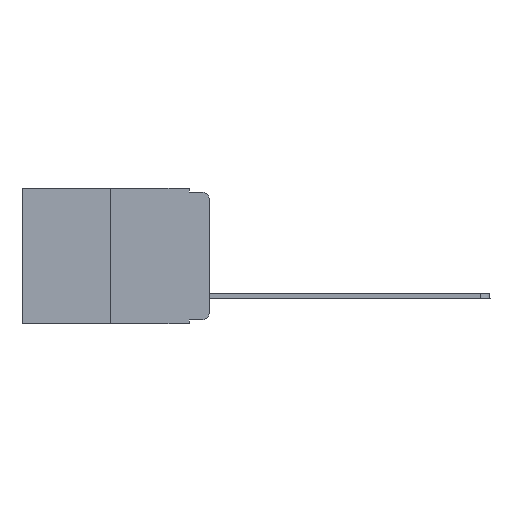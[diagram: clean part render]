
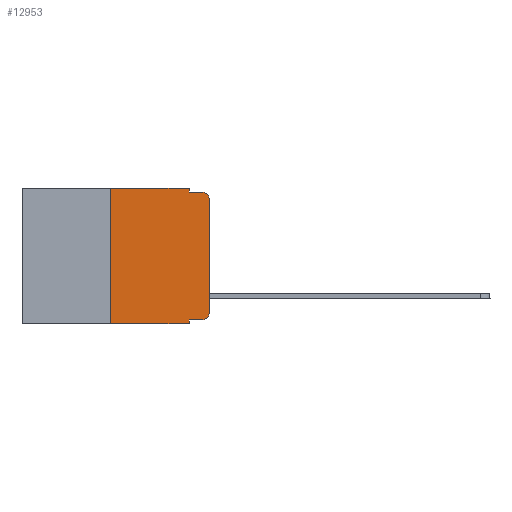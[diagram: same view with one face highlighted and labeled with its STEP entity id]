
A CAD part, left-side view. The second image highlights one B-rep face of the part: STEP entity #12953.
In plain terms, the highlighted planar face has unit normal (-1, 0, 0).
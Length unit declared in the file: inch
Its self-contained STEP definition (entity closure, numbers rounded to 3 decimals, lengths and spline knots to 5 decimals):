
#369 = ORIENTED_EDGE ( 'NONE', *, *, #9170, .F. ) ;
#787 = DIRECTION ( 'NONE',  ( 0., 0., -1. ) ) ;
#1045 = VECTOR ( 'NONE', #8616, 39.37008 ) ;
#1220 = ORIENTED_EDGE ( 'NONE', *, *, #12271, .F. ) ;
#1303 = CARTESIAN_POINT ( 'NONE',  ( 0., 0.02, -0.333 ) ) ;
#1340 = ORIENTED_EDGE ( 'NONE', *, *, #8053, .T. ) ;
#1372 = VERTEX_POINT ( 'NONE', #7355 ) ;
#1584 = CARTESIAN_POINT ( 'NONE',  ( 0., 0.051, 0. ) ) ;
#1749 = DIRECTION ( 'NONE',  ( 0., 0., 1. ) ) ;
#1909 = EDGE_CURVE ( 'NONE', #9740, #6897, #2141, .T. ) ;
#2013 = VERTEX_POINT ( 'NONE', #8496 ) ;
#2141 = LINE ( 'NONE', #3742, #11521 ) ;
#2171 = DIRECTION ( 'NONE',  ( 0., 0., -1. ) ) ;
#2292 = ORIENTED_EDGE ( 'NONE', *, *, #4062, .T. ) ;
#2533 = VECTOR ( 'NONE', #6343, 39.37008 ) ;
#2651 = DIRECTION ( 'NONE',  ( -1., 0., 0. ) ) ;
#2706 = CARTESIAN_POINT ( 'NONE',  ( 0., 0.02, -0.313 ) ) ;
#2746 = VERTEX_POINT ( 'NONE', #13359 ) ;
#2886 = CARTESIAN_POINT ( 'NONE',  ( 0., 0.02, -0.03 ) ) ;
#2942 = LINE ( 'NONE', #5876, #11788 ) ;
#3375 = AXIS2_PLACEMENT_3D ( 'NONE', #2706, #2651, #3918 ) ;
#3420 = AXIS2_PLACEMENT_3D ( 'NONE', #2886, #5226, #787 ) ;
#3734 = VECTOR ( 'NONE', #5573, 39.37008 ) ;
#3742 = CARTESIAN_POINT ( 'NONE',  ( 0., 0.051, 0. ) ) ;
#3799 = DIRECTION ( 'NONE',  ( 0., 0., -1. ) ) ;
#3918 = DIRECTION ( 'NONE',  ( 0., 0., -1. ) ) ;
#4062 = EDGE_CURVE ( 'NONE', #14175, #13535, #10064, .T. ) ;
#4861 = CARTESIAN_POINT ( 'NONE',  ( 0., 0.051, -0.01 ) ) ;
#5122 = VERTEX_POINT ( 'NONE', #8441 ) ;
#5226 = DIRECTION ( 'NONE',  ( -1., 0., 0. ) ) ;
#5497 = LINE ( 'NONE', #12083, #2533 ) ;
#5573 = DIRECTION ( 'NONE',  ( 0., 0., -1. ) ) ;
#5605 = VECTOR ( 'NONE', #13999, 39.37008 ) ;
#5876 = CARTESIAN_POINT ( 'NONE',  ( 0., 0., 0. ) ) ;
#6010 = EDGE_CURVE ( 'NONE', #11974, #1372, #6431, .T. ) ;
#6048 = ORIENTED_EDGE ( 'NONE', *, *, #11104, .T. ) ;
#6094 = EDGE_LOOP ( 'NONE', ( #14177, #1340, #369, #12707, #1220, #8226, #9576, #8156, #6048, #2292 ) ) ;
#6145 = CARTESIAN_POINT ( 'NONE',  ( 0., 0.473, -0.343 ) ) ;
#6343 = DIRECTION ( 'NONE',  ( 0., 0., 1. ) ) ;
#6431 = LINE ( 'NONE', #6145, #1045 ) ;
#6580 = EDGE_CURVE ( 'NONE', #13535, #8024, #2942, .T. ) ;
#6625 = CARTESIAN_POINT ( 'NONE',  ( 0., 0.051, 0. ) ) ;
#6897 = VERTEX_POINT ( 'NONE', #10304 ) ;
#6991 = CARTESIAN_POINT ( 'NONE',  ( 0., 0., -0.03 ) ) ;
#7170 = AXIS2_PLACEMENT_3D ( 'NONE', #8833, #12221, #2171 ) ;
#7210 = VECTOR ( 'NONE', #7667, 39.37008 ) ;
#7355 = CARTESIAN_POINT ( 'NONE',  ( 0., 0.051, -0.343 ) ) ;
#7667 = DIRECTION ( 'NONE',  ( 0., -1., 0. ) ) ;
#7711 = LINE ( 'NONE', #4861, #13931 ) ;
#8024 = VERTEX_POINT ( 'NONE', #6991 ) ;
#8039 = DIRECTION ( 'NONE',  ( 0., -1., 0. ) ) ;
#8053 = EDGE_CURVE ( 'NONE', #8024, #2746, #11399, .T. ) ;
#8156 = ORIENTED_EDGE ( 'NONE', *, *, #12981, .F. ) ;
#8226 = ORIENTED_EDGE ( 'NONE', *, *, #12823, .F. ) ;
#8441 = CARTESIAN_POINT ( 'NONE',  ( 0., 0.25, 0. ) ) ;
#8496 = CARTESIAN_POINT ( 'NONE',  ( 0., 0.051, -0.333 ) ) ;
#8616 = DIRECTION ( 'NONE',  ( 0., -1., 0. ) ) ;
#8833 = CARTESIAN_POINT ( 'NONE',  ( 0., 0.473, 0. ) ) ;
#9124 = LINE ( 'NONE', #6625, #3734 ) ;
#9170 = EDGE_CURVE ( 'NONE', #6897, #2746, #7711, .T. ) ;
#9253 = LINE ( 'NONE', #9574, #5605 ) ;
#9571 = CARTESIAN_POINT ( 'NONE',  ( 0., 0.25, -0.343 ) ) ;
#9574 = CARTESIAN_POINT ( 'NONE',  ( 0., 0.051, -0.333 ) ) ;
#9576 = ORIENTED_EDGE ( 'NONE', *, *, #6010, .T. ) ;
#9740 = VERTEX_POINT ( 'NONE', #1584 ) ;
#10064 = CIRCLE ( 'NONE', #3375, 0.02 ) ;
#10178 = FACE_OUTER_BOUND ( 'NONE', #6094, .T. ) ;
#10304 = CARTESIAN_POINT ( 'NONE',  ( 0., 0.051, -0.01 ) ) ;
#11104 = EDGE_CURVE ( 'NONE', #2013, #14175, #9253, .T. ) ;
#11399 = CIRCLE ( 'NONE', #3420, 0.02 ) ;
#11521 = VECTOR ( 'NONE', #3799, 39.37008 ) ;
#11788 = VECTOR ( 'NONE', #1749, 39.37008 ) ;
#11974 = VERTEX_POINT ( 'NONE', #9571 ) ;
#12083 = CARTESIAN_POINT ( 'NONE',  ( 0., 0.25, 0. ) ) ;
#12115 = CARTESIAN_POINT ( 'NONE',  ( 0., 0., -0.313 ) ) ;
#12129 = PLANE ( 'NONE',  #7170 ) ;
#12221 = DIRECTION ( 'NONE',  ( 1., 0., 0. ) ) ;
#12271 = EDGE_CURVE ( 'NONE', #5122, #9740, #13103, .T. ) ;
#12707 = ORIENTED_EDGE ( 'NONE', *, *, #1909, .F. ) ;
#12823 = EDGE_CURVE ( 'NONE', #11974, #5122, #5497, .T. ) ;
#12953 = ADVANCED_FACE ( 'NONE', ( #10178 ), #12129, .F. ) ;
#12981 = EDGE_CURVE ( 'NONE', #2013, #1372, #9124, .T. ) ;
#13103 = LINE ( 'NONE', #14299, #7210 ) ;
#13359 = CARTESIAN_POINT ( 'NONE',  ( 0., 0.02, -0.01 ) ) ;
#13535 = VERTEX_POINT ( 'NONE', #12115 ) ;
#13931 = VECTOR ( 'NONE', #8039, 39.37008 ) ;
#13999 = DIRECTION ( 'NONE',  ( 0., -1., 0. ) ) ;
#14175 = VERTEX_POINT ( 'NONE', #1303 ) ;
#14177 = ORIENTED_EDGE ( 'NONE', *, *, #6580, .T. ) ;
#14299 = CARTESIAN_POINT ( 'NONE',  ( 0., 0.473, 0. ) ) ;
